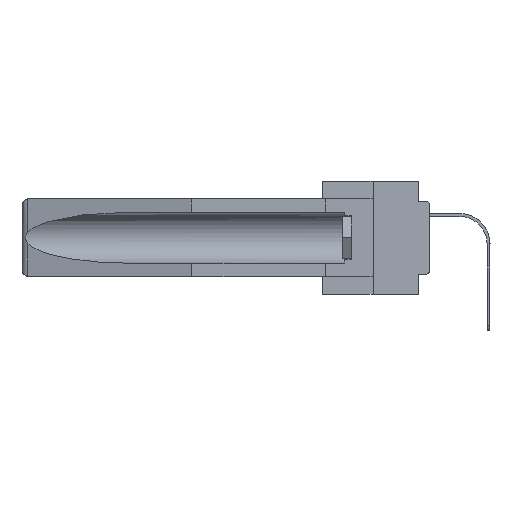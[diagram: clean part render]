
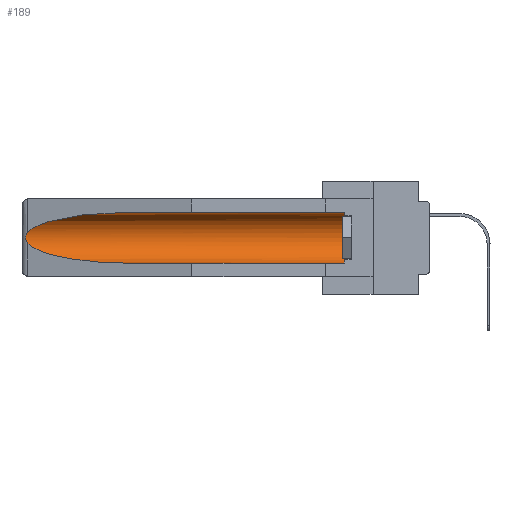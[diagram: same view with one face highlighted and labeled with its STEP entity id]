
A CAD part, left-side view. The second image highlights one B-rep face of the part: STEP entity #189.
In plain terms, the highlighted cylindrical face has radius 2.857 mm (diameter 5.715 mm), a partial arc.
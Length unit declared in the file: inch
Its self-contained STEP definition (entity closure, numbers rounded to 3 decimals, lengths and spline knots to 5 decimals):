
#189 = ADVANCED_FACE ( 'NONE', ( #17824 ), #23650, .F. ) ;
#1363 = CARTESIAN_POINT ( 'NONE',  ( 0.26655, 1.53094, -0.18657 ) ) ;
#2836 = DIRECTION ( 'NONE',  ( 0., 1., 0. ) ) ;
#3288 = VECTOR ( 'NONE', #2836, 39.37008 ) ;
#3489 = LINE ( 'NONE', #14580, #3288 ) ;
#3657 = CARTESIAN_POINT ( 'NONE',  ( 0.2675, 1.53308, -0.16763 ) ) ;
#3884 = ORIENTED_EDGE ( 'NONE', *, *, #7532, .T. ) ;
#4032 = CARTESIAN_POINT ( 'NONE',  ( 0.26537, 1.52718, -0.14972 ) ) ;
#4152 =( BOUNDED_CURVE ( )  B_SPLINE_CURVE ( 3, ( #15473, #23088, #31556, #23267 ),
 .UNSPECIFIED., .F., .F. ) 
 B_SPLINE_CURVE_WITH_KNOTS ( ( 4, 4 ),
 ( 4.71239, 6.08839 ),
 .UNSPECIFIED. ) 
 CURVE ( )  GEOMETRIC_REPRESENTATION_ITEM ( )  RATIONAL_B_SPLINE_CURVE ( ( 1., 0.848, 0.848, 1. ) ) 
 REPRESENTATION_ITEM ( '' )  );
#4640 = CARTESIAN_POINT ( 'NONE',  ( 0.155, 0.126, -0.059 ) ) ;
#4986 = CIRCLE ( 'NONE', #11727, 0.1125 ) ;
#5930 = CARTESIAN_POINT ( 'NONE',  ( 0.26597, 1.52961, -0.15275 ) ) ;
#6039 = CARTESIAN_POINT ( 'NONE',  ( 0.155, 1.07973, -0.059 ) ) ;
#6993 = CARTESIAN_POINT ( 'NONE',  ( 0.21114, 1.30732, -0.284 ) ) ;
#7088 = AXIS2_PLACEMENT_3D ( 'NONE', #21006, #34614, #28600 ) ;
#7532 = EDGE_CURVE ( 'NONE', #12205, #8146, #4152, .T. ) ;
#8146 = VERTEX_POINT ( 'NONE', #4032 ) ;
#9845 = CARTESIAN_POINT ( 'NONE',  ( 0.155, 1.07973, -0.284 ) ) ;
#10026 = CARTESIAN_POINT ( 'NONE',  ( 0.26537, 1.52718, -0.19328 ) ) ;
#11087 = EDGE_CURVE ( 'NONE', #29058, #15378, #4986, .T. ) ;
#11727 = AXIS2_PLACEMENT_3D ( 'NONE', #19542, #19900, #28194 ) ;
#11937 = CARTESIAN_POINT ( 'NONE',  ( 0.155, 1.07973, -0.284 ) ) ;
#12205 = VERTEX_POINT ( 'NONE', #6039 ) ;
#14569 = CARTESIAN_POINT ( 'NONE',  ( 0.26654, 1.53092, -0.15636 ) ) ;
#14580 = CARTESIAN_POINT ( 'NONE',  ( 0.155, -0.30754, -0.284 ) ) ;
#14699 = EDGE_LOOP ( 'NONE', ( #3884, #28882, #30232, #21487, #22393, #25385 ) ) ;
#15378 = VERTEX_POINT ( 'NONE', #4640 ) ;
#15473 = CARTESIAN_POINT ( 'NONE',  ( 0.155, 1.07973, -0.059 ) ) ;
#16810 = EDGE_CURVE ( 'NONE', #27238, #24667, #24675, .T. ) ;
#17824 = FACE_OUTER_BOUND ( 'NONE', #14699, .T. ) ;
#18281 = CARTESIAN_POINT ( 'NONE',  ( 0.155, 0.126, -0.284 ) ) ;
#19264 = DIRECTION ( 'NONE',  ( 0., 1., 0. ) ) ;
#19542 = CARTESIAN_POINT ( 'NONE',  ( 0.155, 0.126, -0.1715 ) ) ;
#19900 = DIRECTION ( 'NONE',  ( 0., -1., 0. ) ) ;
#20062 = CARTESIAN_POINT ( 'NONE',  ( 0.2673, 1.5327, -0.16383 ) ) ;
#21006 = CARTESIAN_POINT ( 'NONE',  ( 0.155, -0.30754, -0.1715 ) ) ;
#21487 = ORIENTED_EDGE ( 'NONE', *, *, #31360, .F. ) ;
#22393 = ORIENTED_EDGE ( 'NONE', *, *, #11087, .T. ) ;
#22435 = LINE ( 'NONE', #32691, #26564 ) ;
#22881 = CARTESIAN_POINT ( 'NONE',  ( 0.2675, 1.53308, -0.17534 ) ) ;
#23088 = CARTESIAN_POINT ( 'NONE',  ( 0.21114, 1.30732, -0.059 ) ) ;
#23267 = CARTESIAN_POINT ( 'NONE',  ( 0.26537, 1.52718, -0.14972 ) ) ;
#23650 = CYLINDRICAL_SURFACE ( 'NONE', #7088, 0.1125 ) ;
#24667 = VERTEX_POINT ( 'NONE', #9845 ) ;
#24675 =( BOUNDED_CURVE ( )  B_SPLINE_CURVE ( 3, ( #34185, #31209, #6993, #11937 ),
 .UNSPECIFIED., .F., .T. ) 
 B_SPLINE_CURVE_WITH_KNOTS ( ( 4, 4 ),
 ( 0.1948, 1.5708 ),
 .UNSPECIFIED. ) 
 CURVE ( )  GEOMETRIC_REPRESENTATION_ITEM ( )  RATIONAL_B_SPLINE_CURVE ( ( 1., 0.848, 0.848, 1. ) ) 
 REPRESENTATION_ITEM ( '' )  );
#25385 = ORIENTED_EDGE ( 'NONE', *, *, #33785, .T. ) ;
#26132 = EDGE_CURVE ( 'NONE', #8146, #27238, #31725, .T. ) ;
#26564 = VECTOR ( 'NONE', #19264, 39.37008 ) ;
#27238 = VERTEX_POINT ( 'NONE', #10026 ) ;
#27666 = CARTESIAN_POINT ( 'NONE',  ( 0.26537, 1.52718, -0.19328 ) ) ;
#28005 = CARTESIAN_POINT ( 'NONE',  ( 0.2673, 1.53269, -0.17917 ) ) ;
#28184 = CARTESIAN_POINT ( 'NONE',  ( 0.26597, 1.5296, -0.19026 ) ) ;
#28194 = DIRECTION ( 'NONE',  ( 0., 0., 1. ) ) ;
#28600 = DIRECTION ( 'NONE',  ( 0., 0., 1. ) ) ;
#28882 = ORIENTED_EDGE ( 'NONE', *, *, #26132, .T. ) ;
#29058 = VERTEX_POINT ( 'NONE', #18281 ) ;
#30232 = ORIENTED_EDGE ( 'NONE', *, *, #16810, .T. ) ;
#31209 = CARTESIAN_POINT ( 'NONE',  ( 0.25451, 1.48313, -0.24835 ) ) ;
#31360 = EDGE_CURVE ( 'NONE', #29058, #24667, #3489, .T. ) ;
#31556 = CARTESIAN_POINT ( 'NONE',  ( 0.25451, 1.48313, -0.09465 ) ) ;
#31725 = B_SPLINE_CURVE_WITH_KNOTS ( 'NONE', 3,
 ( #32104, #5930, #14569, #20062, #3657, #22881, #28005, #1363, #28184, #27666 ),
 .UNSPECIFIED., .F., .F.,
 ( 4, 2, 2, 2, 4 ),
 ( 0., 0.00029, 0.00058, 0.00087, 0.00117 ),
 .UNSPECIFIED. ) ;
#32104 = CARTESIAN_POINT ( 'NONE',  ( 0.26537, 1.52718, -0.14972 ) ) ;
#32691 = CARTESIAN_POINT ( 'NONE',  ( 0.155, -0.30754, -0.059 ) ) ;
#33785 = EDGE_CURVE ( 'NONE', #15378, #12205, #22435, .T. ) ;
#34185 = CARTESIAN_POINT ( 'NONE',  ( 0.26537, 1.52718, -0.19328 ) ) ;
#34614 = DIRECTION ( 'NONE',  ( 0., 1., 0. ) ) ;
